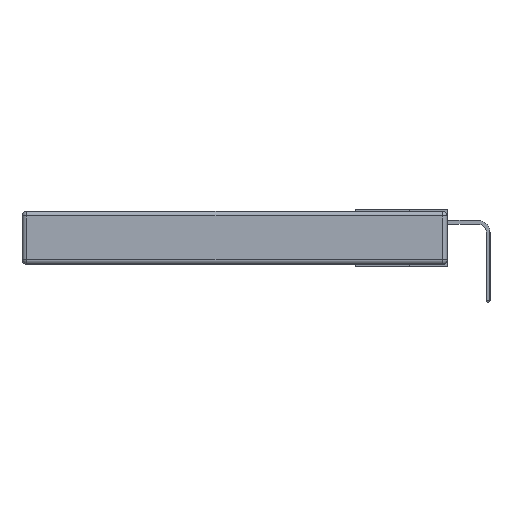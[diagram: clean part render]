
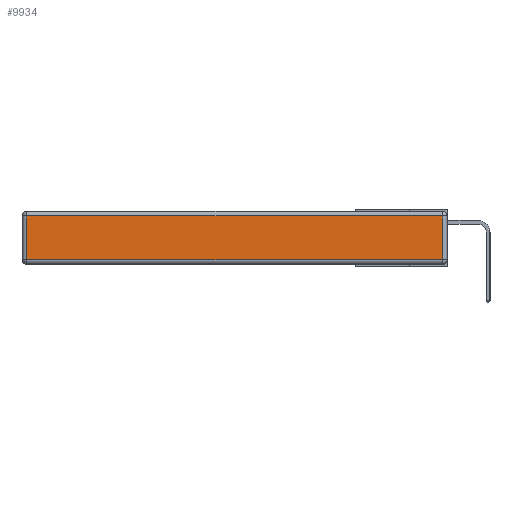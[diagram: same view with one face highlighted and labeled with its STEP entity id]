
A CAD part, left-side view. The second image highlights one B-rep face of the part: STEP entity #9934.
In plain terms, the highlighted planar face has unit normal (-1, 0, 0).
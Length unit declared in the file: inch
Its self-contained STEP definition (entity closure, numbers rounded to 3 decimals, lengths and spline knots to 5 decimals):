
#903 = ORIENTED_EDGE ( 'NONE', *, *, #7487, .T. ) ;
#905 = CARTESIAN_POINT ( 'NONE',  ( 0., 0.03, -0.343 ) ) ;
#1515 = CARTESIAN_POINT ( 'NONE',  ( 0., 2.72, -0.343 ) ) ;
#2129 = CARTESIAN_POINT ( 'NONE',  ( 0., 0., -0.343 ) ) ;
#2197 = CARTESIAN_POINT ( 'NONE',  ( 0., 2.75, -0.03 ) ) ;
#2619 = LINE ( 'NONE', #2197, #14414 ) ;
#3131 = CARTESIAN_POINT ( 'NONE',  ( 0., 0.03, -0.03 ) ) ;
#3190 = DIRECTION ( 'NONE',  ( 0., 0., 1. ) ) ;
#3285 = DIRECTION ( 'NONE',  ( 0., 0., 1. ) ) ;
#3423 = CARTESIAN_POINT ( 'NONE',  ( 0., 0.03, -0.313 ) ) ;
#3636 = CARTESIAN_POINT ( 'NONE',  ( 0., 2.72, -0.313 ) ) ;
#4063 = VERTEX_POINT ( 'NONE', #3131 ) ;
#5163 = FACE_OUTER_BOUND ( 'NONE', #8940, .T. ) ;
#6334 = EDGE_CURVE ( 'NONE', #10246, #4063, #9992, .T. ) ;
#6812 = ORIENTED_EDGE ( 'NONE', *, *, #6334, .T. ) ;
#7487 = EDGE_CURVE ( 'NONE', #14553, #9048, #10861, .T. ) ;
#7628 = VECTOR ( 'NONE', #3190, 39.37008 ) ;
#7679 = VECTOR ( 'NONE', #13981, 39.37008 ) ;
#8940 = EDGE_LOOP ( 'NONE', ( #14010, #6812, #13702, #903 ) ) ;
#9048 = VERTEX_POINT ( 'NONE', #3636 ) ;
#9172 = AXIS2_PLACEMENT_3D ( 'NONE', #2129, #14965, #3285 ) ;
#9685 = LINE ( 'NONE', #11650, #7679 ) ;
#9934 = ADVANCED_FACE ( 'NONE', ( #5163 ), #13828, .T. ) ;
#9992 = LINE ( 'NONE', #905, #7628 ) ;
#10246 = VERTEX_POINT ( 'NONE', #3423 ) ;
#10861 = LINE ( 'NONE', #1515, #13567 ) ;
#10920 = EDGE_CURVE ( 'NONE', #9048, #10246, #9685, .T. ) ;
#11650 = CARTESIAN_POINT ( 'NONE',  ( 0., 0., -0.313 ) ) ;
#11673 = DIRECTION ( 'NONE',  ( 0., 1., 0. ) ) ;
#11998 = DIRECTION ( 'NONE',  ( 0., 0., -1. ) ) ;
#13567 = VECTOR ( 'NONE', #11998, 39.37008 ) ;
#13702 = ORIENTED_EDGE ( 'NONE', *, *, #14937, .T. ) ;
#13828 = PLANE ( 'NONE',  #9172 ) ;
#13981 = DIRECTION ( 'NONE',  ( 0., -1., 0. ) ) ;
#14010 = ORIENTED_EDGE ( 'NONE', *, *, #10920, .T. ) ;
#14210 = CARTESIAN_POINT ( 'NONE',  ( 0., 2.72, -0.03 ) ) ;
#14414 = VECTOR ( 'NONE', #11673, 39.37008 ) ;
#14553 = VERTEX_POINT ( 'NONE', #14210 ) ;
#14937 = EDGE_CURVE ( 'NONE', #4063, #14553, #2619, .T. ) ;
#14965 = DIRECTION ( 'NONE',  ( -1., 0., 0. ) ) ;
